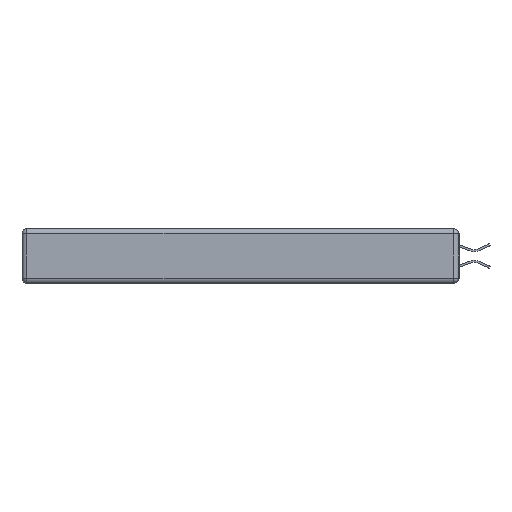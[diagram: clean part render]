
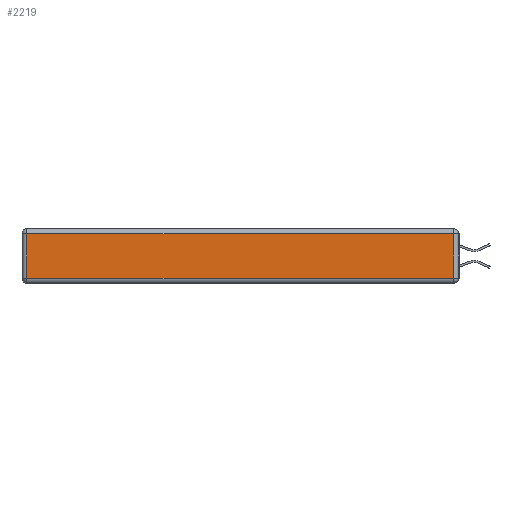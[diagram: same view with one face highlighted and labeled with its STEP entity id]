
A CAD part, left-side view. The second image highlights one B-rep face of the part: STEP entity #2219.
In plain terms, the highlighted planar face has unit normal (-1, 0, 0).
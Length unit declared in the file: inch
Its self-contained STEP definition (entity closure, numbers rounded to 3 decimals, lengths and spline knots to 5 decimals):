
#150 = DIRECTION ( 'NONE',  ( 0., 1., 0. ) ) ;
#228 = EDGE_CURVE ( 'NONE', #6458, #5547, #1696, .T. ) ;
#1396 = CARTESIAN_POINT ( 'NONE',  ( 0., 0.03, -0.313 ) ) ;
#1627 = ORIENTED_EDGE ( 'NONE', *, *, #10897, .T. ) ;
#1696 = LINE ( 'NONE', #8819, #10649 ) ;
#2219 = ADVANCED_FACE ( 'NONE', ( #11913 ), #14814, .T. ) ;
#2225 = ORIENTED_EDGE ( 'NONE', *, *, #7736, .T. ) ;
#2243 = LINE ( 'NONE', #6801, #12754 ) ;
#2923 = VERTEX_POINT ( 'NONE', #3999 ) ;
#3080 = DIRECTION ( 'NONE',  ( 0., -1., 0. ) ) ;
#3168 = VECTOR ( 'NONE', #3208, 39.37008 ) ;
#3208 = DIRECTION ( 'NONE',  ( 0., 0., -1. ) ) ;
#3999 = CARTESIAN_POINT ( 'NONE',  ( 0., 2.72, -0.313 ) ) ;
#4126 = AXIS2_PLACEMENT_3D ( 'NONE', #9899, #7533, #5026 ) ;
#4413 = VERTEX_POINT ( 'NONE', #1396 ) ;
#4764 = ORIENTED_EDGE ( 'NONE', *, *, #5537, .T. ) ;
#5026 = DIRECTION ( 'NONE',  ( 0., 0., 1. ) ) ;
#5537 = EDGE_CURVE ( 'NONE', #5547, #2923, #7165, .T. ) ;
#5547 = VERTEX_POINT ( 'NONE', #11463 ) ;
#6458 = VERTEX_POINT ( 'NONE', #7801 ) ;
#6801 = CARTESIAN_POINT ( 'NONE',  ( 0., 0., -0.313 ) ) ;
#7165 = LINE ( 'NONE', #15455, #3168 ) ;
#7533 = DIRECTION ( 'NONE',  ( -1., 0., 0. ) ) ;
#7736 = EDGE_CURVE ( 'NONE', #4413, #6458, #10702, .T. ) ;
#7801 = CARTESIAN_POINT ( 'NONE',  ( 0., 0.03, -0.03 ) ) ;
#8819 = CARTESIAN_POINT ( 'NONE',  ( 0., 2.75, -0.03 ) ) ;
#9899 = CARTESIAN_POINT ( 'NONE',  ( 0., 0., -0.343 ) ) ;
#10649 = VECTOR ( 'NONE', #150, 39.37008 ) ;
#10702 = LINE ( 'NONE', #13022, #11469 ) ;
#10897 = EDGE_CURVE ( 'NONE', #2923, #4413, #2243, .T. ) ;
#11463 = CARTESIAN_POINT ( 'NONE',  ( 0., 2.72, -0.03 ) ) ;
#11469 = VECTOR ( 'NONE', #14235, 39.37008 ) ;
#11913 = FACE_OUTER_BOUND ( 'NONE', #12723, .T. ) ;
#12723 = EDGE_LOOP ( 'NONE', ( #1627, #2225, #14494, #4764 ) ) ;
#12754 = VECTOR ( 'NONE', #3080, 39.37008 ) ;
#13022 = CARTESIAN_POINT ( 'NONE',  ( 0., 0.03, -0.343 ) ) ;
#14235 = DIRECTION ( 'NONE',  ( 0., 0., 1. ) ) ;
#14494 = ORIENTED_EDGE ( 'NONE', *, *, #228, .T. ) ;
#14814 = PLANE ( 'NONE',  #4126 ) ;
#15455 = CARTESIAN_POINT ( 'NONE',  ( 0., 2.72, -0.343 ) ) ;
